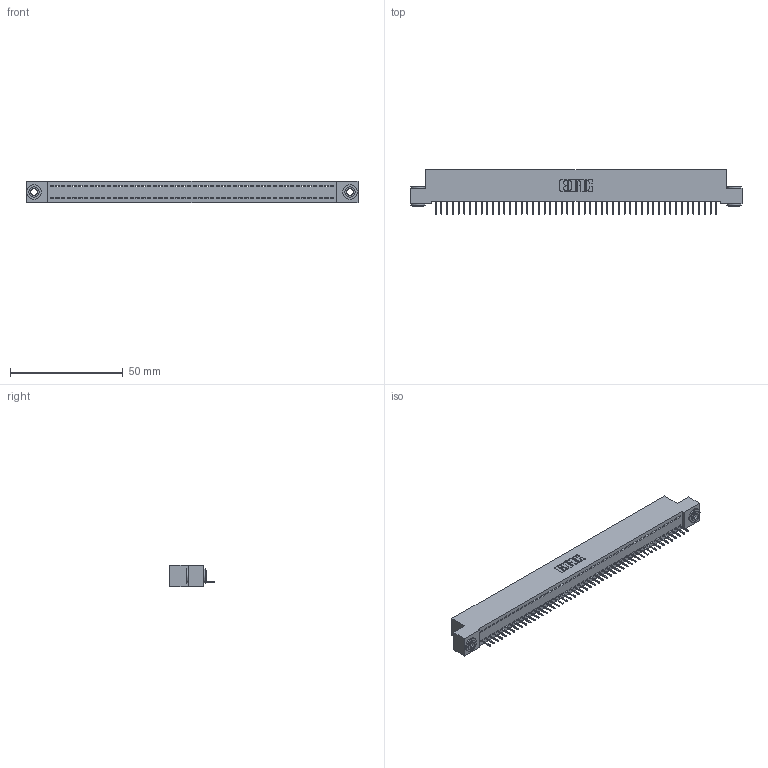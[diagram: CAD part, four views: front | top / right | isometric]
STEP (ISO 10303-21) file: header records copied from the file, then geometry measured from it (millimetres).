
FILE_DESCRIPTION (( 'STEP AP203' ), '1' );
FILE_NAME ('342-050-524-103.STEP', '2018-08-12T19:41:27', ( '' ), ( '' ), 'SwSTEP 2.0', 'SolidWorks 2016', '' );
FILE_SCHEMA (( 'CONFIG_CONTROL_DESIGN' ));
Length unit declared in the file: inch
Products named in the file (4): 342 Part_.156 TH; 345-292-001_345-293-124; 342-250-002_345-250-002-102; 342-050-524-103
Assembly tree (53 placements, depth 2):
  342-050-524-103
    342 Part_.156 TH
    345-292-001_345-293-124  x50
    342-250-002_345-250-002-102  x2
Bounding box: 147.32 x 19.69 x 9.4 mm (x, y, z)
Volume: 12771.8 mm3; surface area: 18516.8 mm2
Topology: 53 solids, 53 shells, 3248 faces, 9375 edges, 6046 vertices
Faces by surface type: plane 2476, cylinder 764, cone 8
Entity records: 30124 total; most frequent: CARTESIAN_POINT 5171, ORIENTED_EDGE 5150, DIRECTION 4381, EDGE_CURVE 2575, VECTOR 2427, LINE 2427, VERTEX_POINT 1710, AXIS2_PLACEMENT_3D 977
